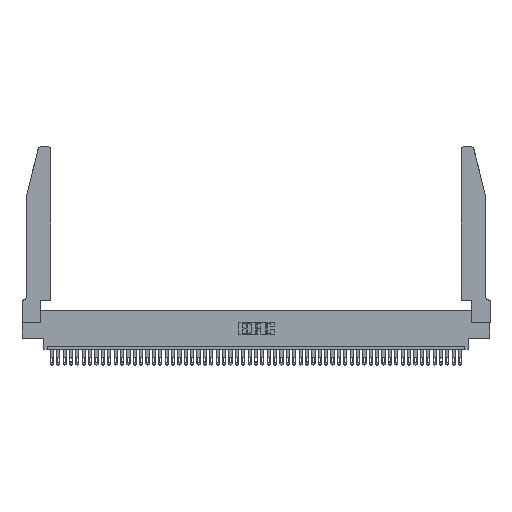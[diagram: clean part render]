
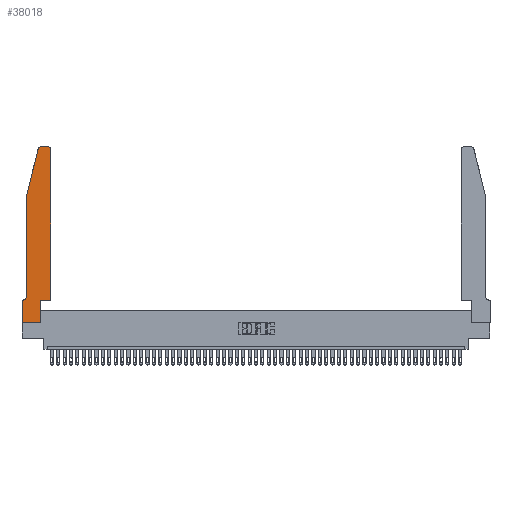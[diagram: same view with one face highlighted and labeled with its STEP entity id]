
A CAD part, top view. The second image highlights one B-rep face of the part: STEP entity #38018.
In plain terms, the highlighted planar face has unit normal (0, 0, 1).
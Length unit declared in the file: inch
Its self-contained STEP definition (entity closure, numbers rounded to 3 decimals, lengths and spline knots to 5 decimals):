
#217 = CARTESIAN_POINT ( 'NONE',  ( 0.4205, 2.72, 0.37 ) ) ;
#581 = AXIS2_PLACEMENT_3D ( 'NONE', #14386, #33478, #33668 ) ;
#865 = LINE ( 'NONE', #15031, #44306 ) ;
#931 = CARTESIAN_POINT ( 'NONE',  ( 0.4505, 0.35, 0.37 ) ) ;
#1016 = DIRECTION ( 'NONE',  ( 0., 1., 0. ) ) ;
#1641 = VERTEX_POINT ( 'NONE', #40411 ) ;
#2114 = AXIS2_PLACEMENT_3D ( 'NONE', #217, #19783, #15992 ) ;
#2201 = DIRECTION ( 'NONE',  ( -0.239, -0.971, 0. ) ) ;
#3715 = LINE ( 'NONE', #9893, #6778 ) ;
#3796 = VERTEX_POINT ( 'NONE', #29609 ) ;
#4660 = VECTOR ( 'NONE', #5808, 39.37008 ) ;
#4924 = CIRCLE ( 'NONE', #45220, 0.03 ) ;
#5548 = ORIENTED_EDGE ( 'NONE', *, *, #27987, .T. ) ;
#5808 = DIRECTION ( 'NONE',  ( -1., 0., 0. ) ) ;
#6608 = LINE ( 'NONE', #45595, #26164 ) ;
#6676 = CARTESIAN_POINT ( 'NONE',  ( 0., 0.35, 0.37 ) ) ;
#6778 = VECTOR ( 'NONE', #2201, 39.37008 ) ;
#7162 = ORIENTED_EDGE ( 'NONE', *, *, #23229, .T. ) ;
#8329 = CARTESIAN_POINT ( 'NONE',  ( 0.4505, 2.72, 0.37 ) ) ;
#8657 = CARTESIAN_POINT ( 'NONE',  ( 0., 0., 0.37 ) ) ;
#9525 = CARTESIAN_POINT ( 'NONE',  ( 0.25487, 2.72718, 0.37 ) ) ;
#9893 = CARTESIAN_POINT ( 'NONE',  ( 0.0755, 2., 0.37 ) ) ;
#9942 = DIRECTION ( 'NONE',  ( 0., 0., 1. ) ) ;
#10392 = ORIENTED_EDGE ( 'NONE', *, *, #12257, .T. ) ;
#10437 = EDGE_CURVE ( 'NONE', #49687, #3796, #30451, .T. ) ;
#11095 = DIRECTION ( 'NONE',  ( 1., 0., 0. ) ) ;
#11794 = DIRECTION ( 'NONE',  ( 1., 0., 0. ) ) ;
#12154 = CARTESIAN_POINT ( 'NONE',  ( 0.2865, 0., 0.37 ) ) ;
#12257 = EDGE_CURVE ( 'NONE', #22698, #26760, #3715, .T. ) ;
#13421 = DIRECTION ( 'NONE',  ( -1., 0., 0. ) ) ;
#13903 = CARTESIAN_POINT ( 'NONE',  ( 0.0755, 0.35, 0.37 ) ) ;
#14386 = CARTESIAN_POINT ( 'NONE',  ( 0.0055, 0.42, 0.37 ) ) ;
#14719 = EDGE_CURVE ( 'NONE', #1641, #39048, #17608, .T. ) ;
#14838 = CARTESIAN_POINT ( 'NONE',  ( 0.0755, 2., 0.37 ) ) ;
#14964 = ORIENTED_EDGE ( 'NONE', *, *, #40453, .T. ) ;
#15031 = CARTESIAN_POINT ( 'NONE',  ( 0., 0., 0.37 ) ) ;
#15410 = CARTESIAN_POINT ( 'NONE',  ( 0.4505, 0.35, 0.37 ) ) ;
#15992 = DIRECTION ( 'NONE',  ( 1., 0., 0. ) ) ;
#17486 = CARTESIAN_POINT ( 'NONE',  ( 0.4205, 2.75, 0.37 ) ) ;
#17608 = CIRCLE ( 'NONE', #581, 0.07 ) ;
#18011 = PLANE ( 'NONE',  #45809 ) ;
#19783 = DIRECTION ( 'NONE',  ( 0., 0., 1. ) ) ;
#20180 = VERTEX_POINT ( 'NONE', #25391 ) ;
#20700 = CARTESIAN_POINT ( 'NONE',  ( 0.2865, 0.35, 0.37 ) ) ;
#21097 = EDGE_CURVE ( 'NONE', #40065, #34053, #29302, .T. ) ;
#21268 = CARTESIAN_POINT ( 'NONE',  ( 0.2605, 2.75, 0.37 ) ) ;
#21680 = EDGE_CURVE ( 'NONE', #20180, #26540, #6608, .T. ) ;
#21824 = CARTESIAN_POINT ( 'NONE',  ( 0.0755, 2., 0.37 ) ) ;
#22258 = VECTOR ( 'NONE', #13421, 39.37008 ) ;
#22548 = CARTESIAN_POINT ( 'NONE',  ( 0.284, 2.72, 0.37 ) ) ;
#22698 = VERTEX_POINT ( 'NONE', #9525 ) ;
#23035 = DIRECTION ( 'NONE',  ( 0., 0., 1. ) ) ;
#23229 = EDGE_CURVE ( 'NONE', #26540, #49687, #865, .T. ) ;
#24449 = DIRECTION ( 'NONE',  ( 1., 0., 0. ) ) ;
#24538 = LINE ( 'NONE', #24947, #25771 ) ;
#24947 = CARTESIAN_POINT ( 'NONE',  ( 0.4505, 0.35, 0.37 ) ) ;
#25154 = ORIENTED_EDGE ( 'NONE', *, *, #21680, .T. ) ;
#25391 = CARTESIAN_POINT ( 'NONE',  ( 0., 0.35, 0.37 ) ) ;
#25771 = VECTOR ( 'NONE', #24449, 39.37008 ) ;
#25775 = ORIENTED_EDGE ( 'NONE', *, *, #29695, .T. ) ;
#26164 = VECTOR ( 'NONE', #38461, 39.37008 ) ;
#26540 = VERTEX_POINT ( 'NONE', #8657 ) ;
#26760 = VERTEX_POINT ( 'NONE', #21824 ) ;
#27077 = ORIENTED_EDGE ( 'NONE', *, *, #36953, .T. ) ;
#27669 = ORIENTED_EDGE ( 'NONE', *, *, #21097, .T. ) ;
#27987 = EDGE_CURVE ( 'NONE', #3796, #40065, #24538, .T. ) ;
#29302 = LINE ( 'NONE', #931, #37230 ) ;
#29609 = CARTESIAN_POINT ( 'NONE',  ( 0.2865, 0.35, 0.37 ) ) ;
#29695 = EDGE_CURVE ( 'NONE', #49258, #33359, #31383, .T. ) ;
#29704 = DIRECTION ( 'NONE',  ( 0., -1., 0. ) ) ;
#30451 = LINE ( 'NONE', #20700, #39644 ) ;
#31383 = LINE ( 'NONE', #21268, #22258 ) ;
#33076 = CARTESIAN_POINT ( 'NONE',  ( 0.0055, 0.35, 0.37 ) ) ;
#33359 = VERTEX_POINT ( 'NONE', #48889 ) ;
#33478 = DIRECTION ( 'NONE',  ( 0., 0., -1. ) ) ;
#33668 = DIRECTION ( 'NONE',  ( -1., 0., 0. ) ) ;
#34030 = DIRECTION ( 'NONE',  ( 1., 0., 0. ) ) ;
#34053 = VERTEX_POINT ( 'NONE', #8329 ) ;
#34432 = EDGE_CURVE ( 'NONE', #26760, #1641, #36414, .T. ) ;
#35464 = ORIENTED_EDGE ( 'NONE', *, *, #34432, .T. ) ;
#35810 = DIRECTION ( 'NONE',  ( 0., 1., 0. ) ) ;
#36414 = LINE ( 'NONE', #14838, #47358 ) ;
#36953 = EDGE_CURVE ( 'NONE', #39048, #20180, #37782, .T. ) ;
#37211 = EDGE_LOOP ( 'NONE', ( #25775, #14964, #10392, #35464, #47027, #27077, #25154, #7162, #39671, #5548, #27669, #44007 ) ) ;
#37230 = VECTOR ( 'NONE', #35810, 39.37008 ) ;
#37782 = LINE ( 'NONE', #13903, #4660 ) ;
#38018 = ADVANCED_FACE ( 'NONE', ( #50427 ), #18011, .T. ) ;
#38461 = DIRECTION ( 'NONE',  ( 0., -1., 0. ) ) ;
#39048 = VERTEX_POINT ( 'NONE', #33076 ) ;
#39644 = VECTOR ( 'NONE', #1016, 39.37008 ) ;
#39671 = ORIENTED_EDGE ( 'NONE', *, *, #10437, .T. ) ;
#40065 = VERTEX_POINT ( 'NONE', #15410 ) ;
#40411 = CARTESIAN_POINT ( 'NONE',  ( 0.0755, 0.42, 0.37 ) ) ;
#40453 = EDGE_CURVE ( 'NONE', #33359, #22698, #4924, .T. ) ;
#43825 = CIRCLE ( 'NONE', #2114, 0.03 ) ;
#44007 = ORIENTED_EDGE ( 'NONE', *, *, #44478, .T. ) ;
#44306 = VECTOR ( 'NONE', #11794, 39.37008 ) ;
#44478 = EDGE_CURVE ( 'NONE', #34053, #49258, #43825, .T. ) ;
#45220 = AXIS2_PLACEMENT_3D ( 'NONE', #22548, #23035, #11095 ) ;
#45595 = CARTESIAN_POINT ( 'NONE',  ( 0., 0., 0.37 ) ) ;
#45809 = AXIS2_PLACEMENT_3D ( 'NONE', #6676, #9942, #34030 ) ;
#47027 = ORIENTED_EDGE ( 'NONE', *, *, #14719, .T. ) ;
#47358 = VECTOR ( 'NONE', #29704, 39.37008 ) ;
#48889 = CARTESIAN_POINT ( 'NONE',  ( 0.284, 2.75, 0.37 ) ) ;
#49258 = VERTEX_POINT ( 'NONE', #17486 ) ;
#49687 = VERTEX_POINT ( 'NONE', #12154 ) ;
#50427 = FACE_OUTER_BOUND ( 'NONE', #37211, .T. ) ;
